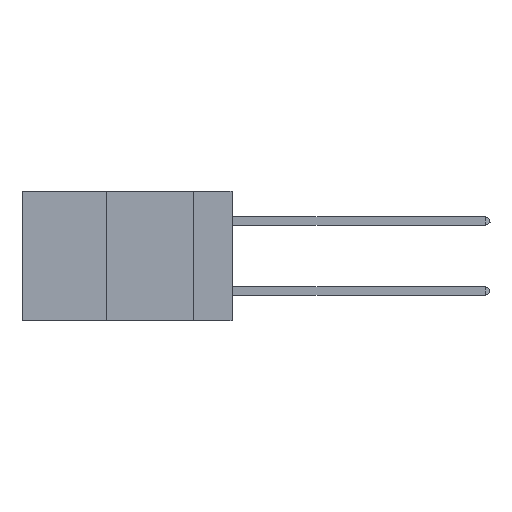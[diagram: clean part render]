
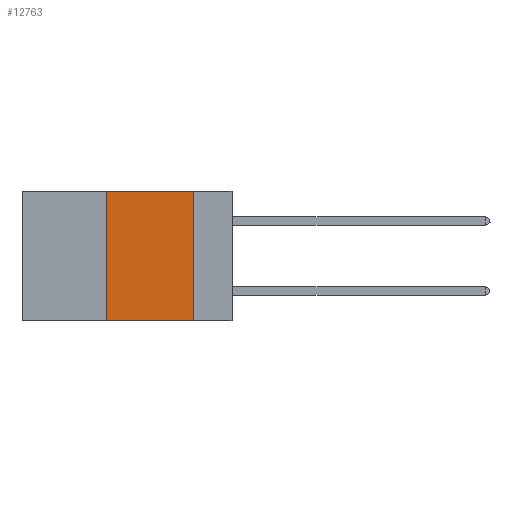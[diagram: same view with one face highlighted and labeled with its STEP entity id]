
A CAD part, left-side view. The second image highlights one B-rep face of the part: STEP entity #12763.
In plain terms, the highlighted planar face has unit normal (-1, 0, 0).
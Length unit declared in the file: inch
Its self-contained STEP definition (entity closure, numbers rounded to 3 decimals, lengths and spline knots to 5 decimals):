
#375 = VECTOR ( 'NONE', #853, 39.37008 ) ;
#516 = PLANE ( 'NONE',  #10309 ) ;
#853 = DIRECTION ( 'NONE',  ( 0., 0., -1. ) ) ;
#1055 = VECTOR ( 'NONE', #16773, 39.37008 ) ;
#1419 = CARTESIAN_POINT ( 'NONE',  ( 0., 0.36, -0.37 ) ) ;
#1958 = CARTESIAN_POINT ( 'NONE',  ( 0., 0.6, 0. ) ) ;
#2312 = LINE ( 'NONE', #4171, #7208 ) ;
#2709 = ORIENTED_EDGE ( 'NONE', *, *, #3012, .T. ) ;
#3012 = EDGE_CURVE ( 'NONE', #15350, #5710, #19887, .T. ) ;
#4066 = LINE ( 'NONE', #4379, #375 ) ;
#4171 = CARTESIAN_POINT ( 'NONE',  ( 0., 0.6, 0. ) ) ;
#4246 = EDGE_LOOP ( 'NONE', ( #17891, #11795, #8933, #2709 ) ) ;
#4379 = CARTESIAN_POINT ( 'NONE',  ( 0., 0.11, 0. ) ) ;
#5710 = VERTEX_POINT ( 'NONE', #15018 ) ;
#6453 = DIRECTION ( 'NONE',  ( 0., 0., 1. ) ) ;
#7089 = CARTESIAN_POINT ( 'NONE',  ( 0., 0.6, -0.37 ) ) ;
#7208 = VECTOR ( 'NONE', #16664, 39.37008 ) ;
#7669 = EDGE_CURVE ( 'NONE', #15350, #18351, #12704, .T. ) ;
#8933 = ORIENTED_EDGE ( 'NONE', *, *, #7669, .F. ) ;
#10309 = AXIS2_PLACEMENT_3D ( 'NONE', #1958, #16299, #19434 ) ;
#10842 = CARTESIAN_POINT ( 'NONE',  ( 0., 0.11, 0. ) ) ;
#10930 = VERTEX_POINT ( 'NONE', #10842 ) ;
#11795 = ORIENTED_EDGE ( 'NONE', *, *, #16097, .F. ) ;
#12704 = LINE ( 'NONE', #12804, #18682 ) ;
#12763 = ADVANCED_FACE ( 'NONE', ( #12975 ), #516, .F. ) ;
#12804 = CARTESIAN_POINT ( 'NONE',  ( 0., 0.36, 0. ) ) ;
#12975 = FACE_OUTER_BOUND ( 'NONE', #4246, .T. ) ;
#13014 = EDGE_CURVE ( 'NONE', #10930, #5710, #4066, .T. ) ;
#15018 = CARTESIAN_POINT ( 'NONE',  ( 0., 0.11, -0.37 ) ) ;
#15350 = VERTEX_POINT ( 'NONE', #1419 ) ;
#16097 = EDGE_CURVE ( 'NONE', #18351, #10930, #2312, .T. ) ;
#16299 = DIRECTION ( 'NONE',  ( 1., 0., 0. ) ) ;
#16664 = DIRECTION ( 'NONE',  ( 0., -1., 0. ) ) ;
#16773 = DIRECTION ( 'NONE',  ( 0., -1., 0. ) ) ;
#17891 = ORIENTED_EDGE ( 'NONE', *, *, #13014, .F. ) ;
#18351 = VERTEX_POINT ( 'NONE', #18829 ) ;
#18682 = VECTOR ( 'NONE', #6453, 39.37008 ) ;
#18829 = CARTESIAN_POINT ( 'NONE',  ( 0., 0.36, 0. ) ) ;
#19434 = DIRECTION ( 'NONE',  ( 0., 0., -1. ) ) ;
#19887 = LINE ( 'NONE', #7089, #1055 ) ;
